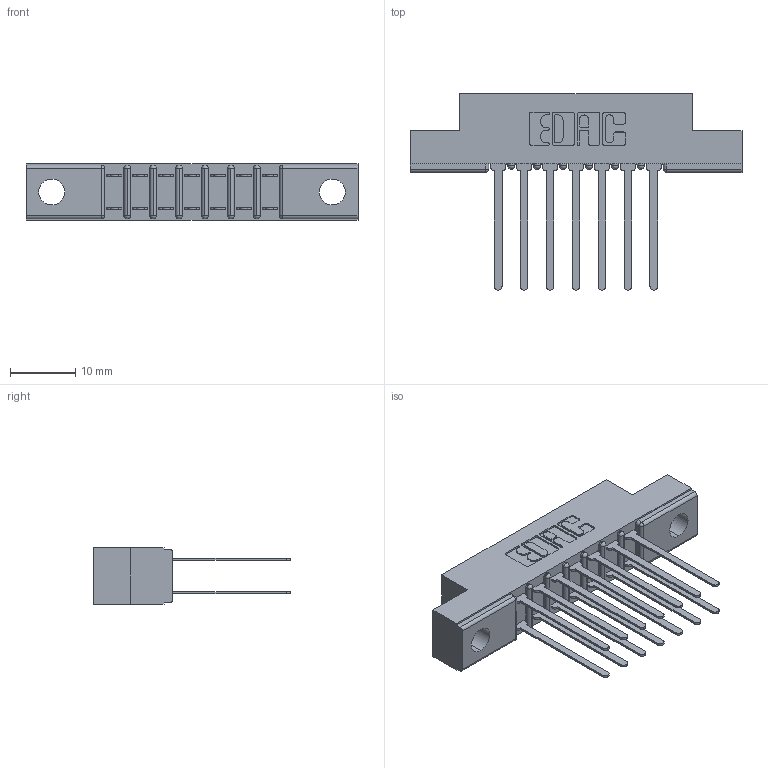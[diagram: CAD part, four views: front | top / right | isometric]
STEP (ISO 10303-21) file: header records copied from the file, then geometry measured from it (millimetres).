
FILE_DESCRIPTION (( 'STEP AP203' ), '1' );
FILE_NAME ('307-014-440-204.STEP', '2020-09-28T15:52:13', ( '' ), ( '' ), 'SwSTEP 2.0', 'SolidWorks 2020', '' );
FILE_SCHEMA (( 'CONFIG_CONTROL_DESIGN' ));
Length unit declared in the file: inch
Products named in the file (3): 307-014-440-204; 307 Part_.156 Dia Mounting Holes; 307-290-001_540
Assembly tree (15 placements, depth 2):
  307-014-440-204
    307 Part_.156 Dia Mounting Holes
    307-290-001_540  x14
Bounding box: 50.75 x 30 x 8.71 mm (x, y, z)
Volume: 3293.4 mm3; surface area: 5369.3 mm2
Topology: 15 solids, 15 shells, 784 faces, 2179 edges, 1410 vertices
Faces by surface type: plane 518, cylinder 250, sphere 16
Entity records: 10926 total; most frequent: CARTESIAN_POINT 1801, ORIENTED_EDGE 1778, DIRECTION 1771, EDGE_CURVE 889, LINE 675, VECTOR 675, VERTEX_POINT 578, AXIS2_PLACEMENT_3D 548
